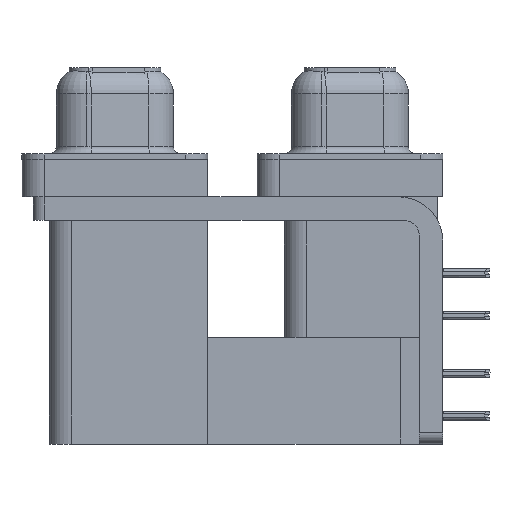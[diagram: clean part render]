
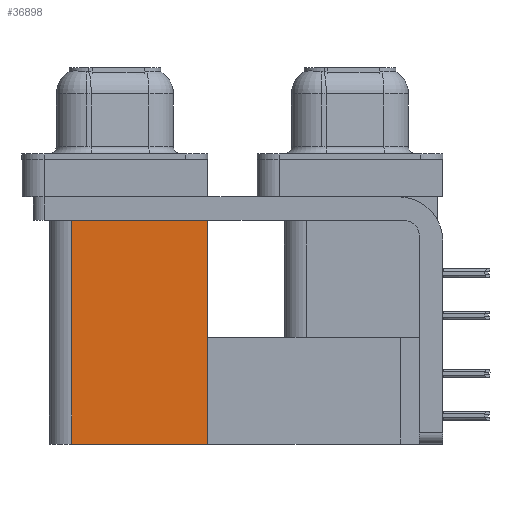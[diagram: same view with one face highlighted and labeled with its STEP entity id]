
A CAD part, left-side view. The second image highlights one B-rep face of the part: STEP entity #36898.
In plain terms, the highlighted planar face has unit normal (-1, 0, 0).
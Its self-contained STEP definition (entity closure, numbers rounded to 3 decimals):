
#86 = EDGE_LOOP ( 'NONE', ( #3294, #4563, #42247, #24591 ) ) ;
#1709 = CARTESIAN_POINT ( 'NONE',  ( 3.765, 9.6, -19.2 ) ) ;
#2533 = AXIS2_PLACEMENT_3D ( 'NONE', #1709, #4926, #8860 ) ;
#2632 = VECTOR ( 'NONE', #11673, 1000. ) ;
#3294 = ORIENTED_EDGE ( 'NONE', *, *, #34578, .T. ) ;
#4379 = EDGE_CURVE ( 'NONE', #33741, #25197, #38305, .T. ) ;
#4425 = DIRECTION ( 'NONE',  ( 0., 1., 0. ) ) ;
#4563 = ORIENTED_EDGE ( 'NONE', *, *, #40295, .F. ) ;
#4718 = VECTOR ( 'NONE', #31826, 1000. ) ;
#4926 = DIRECTION ( 'NONE',  ( 1., 0., 0. ) ) ;
#8860 = DIRECTION ( 'NONE',  ( 0., 0., -1. ) ) ;
#10703 = CARTESIAN_POINT ( 'NONE',  ( 3.765, 18.8, -2.5 ) ) ;
#11421 = LINE ( 'NONE', #41593, #2632 ) ;
#11673 = DIRECTION ( 'NONE',  ( 0., 0., 1. ) ) ;
#13010 = VERTEX_POINT ( 'NONE', #17248 ) ;
#13057 = CARTESIAN_POINT ( 'NONE',  ( 3.765, 9.6, -2.5 ) ) ;
#16424 = VECTOR ( 'NONE', #28411, 1000. ) ;
#17248 = CARTESIAN_POINT ( 'NONE',  ( 3.765, 9.6, -2.5 ) ) ;
#18853 = VERTEX_POINT ( 'NONE', #10703 ) ;
#20452 = LINE ( 'NONE', #35545, #4718 ) ;
#20974 = LINE ( 'NONE', #13057, #16424 ) ;
#23218 = CARTESIAN_POINT ( 'NONE',  ( 3.765, 9.6, -19.2 ) ) ;
#23740 = CARTESIAN_POINT ( 'NONE',  ( 3.765, 18.8, -19.2 ) ) ;
#24591 = ORIENTED_EDGE ( 'NONE', *, *, #43690, .T. ) ;
#25197 = VERTEX_POINT ( 'NONE', #23740 ) ;
#28411 = DIRECTION ( 'NONE',  ( 0., 1., 0. ) ) ;
#31120 = PLANE ( 'NONE',  #2533 ) ;
#31826 = DIRECTION ( 'NONE',  ( 0., 0., 1. ) ) ;
#33741 = VERTEX_POINT ( 'NONE', #48367 ) ;
#34578 = EDGE_CURVE ( 'NONE', #13010, #18853, #20974, .T. ) ;
#35545 = CARTESIAN_POINT ( 'NONE',  ( 3.765, 9.6, -19.2 ) ) ;
#36898 = ADVANCED_FACE ( 'NONE', ( #42977 ), #31120, .F. ) ;
#36919 = VECTOR ( 'NONE', #4425, 1000. ) ;
#38305 = LINE ( 'NONE', #23218, #36919 ) ;
#40295 = EDGE_CURVE ( 'NONE', #25197, #18853, #11421, .T. ) ;
#41593 = CARTESIAN_POINT ( 'NONE',  ( 3.765, 18.8, -19.2 ) ) ;
#42247 = ORIENTED_EDGE ( 'NONE', *, *, #4379, .F. ) ;
#42977 = FACE_OUTER_BOUND ( 'NONE', #86, .T. ) ;
#43690 = EDGE_CURVE ( 'NONE', #33741, #13010, #20452, .T. ) ;
#48367 = CARTESIAN_POINT ( 'NONE',  ( 3.765, 9.6, -19.2 ) ) ;
